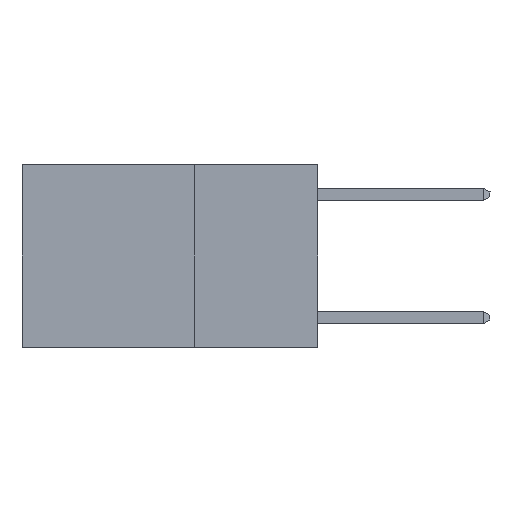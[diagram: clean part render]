
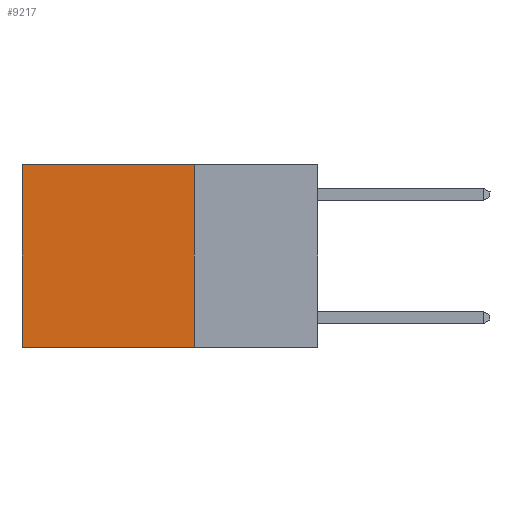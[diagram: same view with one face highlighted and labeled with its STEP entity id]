
A CAD part, left-side view. The second image highlights one B-rep face of the part: STEP entity #9217.
In plain terms, the highlighted planar face has unit normal (-1, 0, 0).
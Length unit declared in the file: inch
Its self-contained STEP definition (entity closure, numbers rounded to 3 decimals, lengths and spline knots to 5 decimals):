
#963 = FACE_OUTER_BOUND ( 'NONE', #11664, .T. ) ;
#1685 = ORIENTED_EDGE ( 'NONE', *, *, #12335, .F. ) ;
#1859 = CARTESIAN_POINT ( 'NONE',  ( 0.2625, 0.25, 0. ) ) ;
#1890 = CARTESIAN_POINT ( 'NONE',  ( 0.2625, 0.25, -0.37 ) ) ;
#2202 = DIRECTION ( 'NONE',  ( 1., 0., 0. ) ) ;
#2247 = VECTOR ( 'NONE', #12565, 39.37008 ) ;
#2454 = EDGE_CURVE ( 'NONE', #5914, #8449, #6184, .T. ) ;
#2536 = CARTESIAN_POINT ( 'NONE',  ( 0.2625, 0.25, -0.37 ) ) ;
#2718 = ORIENTED_EDGE ( 'NONE', *, *, #9200, .T. ) ;
#3008 = ORIENTED_EDGE ( 'NONE', *, *, #9824, .F. ) ;
#4275 = VERTEX_POINT ( 'NONE', #7253 ) ;
#4344 = VECTOR ( 'NONE', #7131, 39.37008 ) ;
#5914 = VERTEX_POINT ( 'NONE', #7682 ) ;
#6184 = LINE ( 'NONE', #9466, #2247 ) ;
#6370 = DIRECTION ( 'NONE',  ( 0., 0., -1. ) ) ;
#6561 = VECTOR ( 'NONE', #6370, 39.37008 ) ;
#7131 = DIRECTION ( 'NONE',  ( 0., 1., 0. ) ) ;
#7253 = CARTESIAN_POINT ( 'NONE',  ( 0.2625, 0.6, -0.37 ) ) ;
#7384 = VECTOR ( 'NONE', #9235, 39.37008 ) ;
#7438 = PLANE ( 'NONE',  #9213 ) ;
#7682 = CARTESIAN_POINT ( 'NONE',  ( 0.2625, 0.25, 0. ) ) ;
#8449 = VERTEX_POINT ( 'NONE', #11459 ) ;
#8506 = CARTESIAN_POINT ( 'NONE',  ( 0.2625, 0.25, 0. ) ) ;
#9200 = EDGE_CURVE ( 'NONE', #8449, #4275, #9391, .T. ) ;
#9213 = AXIS2_PLACEMENT_3D ( 'NONE', #8506, #2202, #9566 ) ;
#9217 = ADVANCED_FACE ( 'NONE', ( #963 ), #7438, .F. ) ;
#9235 = DIRECTION ( 'NONE',  ( 0., 0., -1. ) ) ;
#9391 = LINE ( 'NONE', #10570, #6561 ) ;
#9466 = CARTESIAN_POINT ( 'NONE',  ( 0.2625, 0.25, 0. ) ) ;
#9566 = DIRECTION ( 'NONE',  ( 0., 0., -1. ) ) ;
#9824 = EDGE_CURVE ( 'NONE', #5914, #12052, #12963, .T. ) ;
#9946 = LINE ( 'NONE', #1890, #4344 ) ;
#10570 = CARTESIAN_POINT ( 'NONE',  ( 0.2625, 0.6, 0. ) ) ;
#11459 = CARTESIAN_POINT ( 'NONE',  ( 0.2625, 0.6, 0. ) ) ;
#11664 = EDGE_LOOP ( 'NONE', ( #2718, #1685, #3008, #13566 ) ) ;
#12052 = VERTEX_POINT ( 'NONE', #2536 ) ;
#12335 = EDGE_CURVE ( 'NONE', #12052, #4275, #9946, .T. ) ;
#12565 = DIRECTION ( 'NONE',  ( 0., 1., 0. ) ) ;
#12963 = LINE ( 'NONE', #1859, #7384 ) ;
#13566 = ORIENTED_EDGE ( 'NONE', *, *, #2454, .T. ) ;
